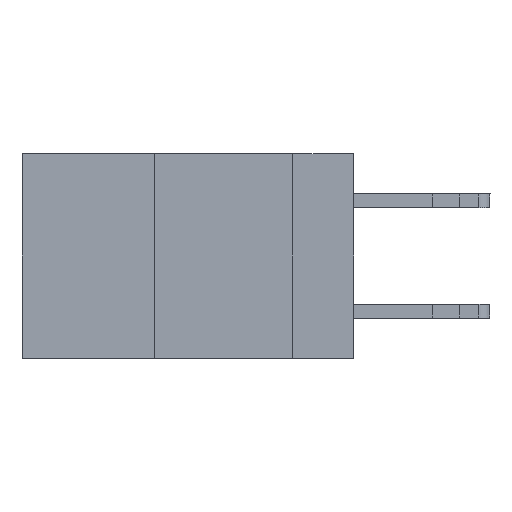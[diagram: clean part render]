
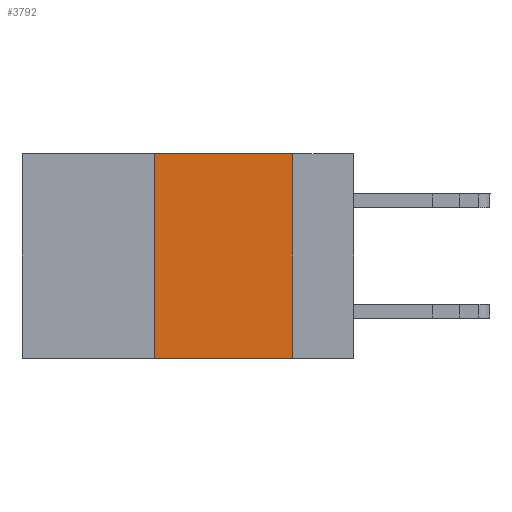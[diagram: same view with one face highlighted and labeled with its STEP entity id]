
A CAD part, left-side view. The second image highlights one B-rep face of the part: STEP entity #3792.
In plain terms, the highlighted planar face has unit normal (-1, 0, 0).
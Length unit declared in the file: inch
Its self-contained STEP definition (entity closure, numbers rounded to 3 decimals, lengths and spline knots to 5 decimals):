
#47 = ORIENTED_EDGE ( 'NONE', *, *, #14907, .T. ) ;
#554 = CARTESIAN_POINT ( 'NONE',  ( 0., 0.36, -0.37 ) ) ;
#1004 = CARTESIAN_POINT ( 'NONE',  ( 0., 0.6, -0.37 ) ) ;
#1065 = VECTOR ( 'NONE', #13622, 39.37008 ) ;
#1487 = DIRECTION ( 'NONE',  ( 0., -1., 0. ) ) ;
#2395 = CARTESIAN_POINT ( 'NONE',  ( 0., 0.6, 0. ) ) ;
#2685 = FACE_OUTER_BOUND ( 'NONE', #14182, .T. ) ;
#3030 = EDGE_CURVE ( 'NONE', #3723, #9920, #15404, .T. ) ;
#3723 = VERTEX_POINT ( 'NONE', #554 ) ;
#3792 = ADVANCED_FACE ( 'NONE', ( #2685 ), #3929, .F. ) ;
#3929 = PLANE ( 'NONE',  #10517 ) ;
#4660 = ORIENTED_EDGE ( 'NONE', *, *, #3030, .F. ) ;
#4810 = LINE ( 'NONE', #5394, #9489 ) ;
#5394 = CARTESIAN_POINT ( 'NONE',  ( 0., 0.11, 0. ) ) ;
#5586 = DIRECTION ( 'NONE',  ( 0., 0., -1. ) ) ;
#7175 = DIRECTION ( 'NONE',  ( 1., 0., 0. ) ) ;
#8979 = CARTESIAN_POINT ( 'NONE',  ( 0., 0.36, 0. ) ) ;
#9489 = VECTOR ( 'NONE', #19472, 39.37008 ) ;
#9553 = EDGE_CURVE ( 'NONE', #17729, #17404, #4810, .T. ) ;
#9920 = VERTEX_POINT ( 'NONE', #19717 ) ;
#10517 = AXIS2_PLACEMENT_3D ( 'NONE', #2395, #7175, #5586 ) ;
#11142 = VECTOR ( 'NONE', #15191, 39.37008 ) ;
#12611 = CARTESIAN_POINT ( 'NONE',  ( 0., 0.6, 0. ) ) ;
#13219 = EDGE_CURVE ( 'NONE', #9920, #17729, #15350, .T. ) ;
#13622 = DIRECTION ( 'NONE',  ( 0., -1., 0. ) ) ;
#14182 = EDGE_LOOP ( 'NONE', ( #15876, #19335, #4660, #47 ) ) ;
#14536 = CARTESIAN_POINT ( 'NONE',  ( 0., 0.11, 0. ) ) ;
#14902 = CARTESIAN_POINT ( 'NONE',  ( 0., 0.11, -0.37 ) ) ;
#14907 = EDGE_CURVE ( 'NONE', #3723, #17404, #18219, .T. ) ;
#15191 = DIRECTION ( 'NONE',  ( 0., 0., 1. ) ) ;
#15350 = LINE ( 'NONE', #12611, #19290 ) ;
#15404 = LINE ( 'NONE', #8979, #11142 ) ;
#15876 = ORIENTED_EDGE ( 'NONE', *, *, #9553, .F. ) ;
#17404 = VERTEX_POINT ( 'NONE', #14902 ) ;
#17729 = VERTEX_POINT ( 'NONE', #14536 ) ;
#18219 = LINE ( 'NONE', #1004, #1065 ) ;
#19290 = VECTOR ( 'NONE', #1487, 39.37008 ) ;
#19335 = ORIENTED_EDGE ( 'NONE', *, *, #13219, .F. ) ;
#19472 = DIRECTION ( 'NONE',  ( 0., 0., -1. ) ) ;
#19717 = CARTESIAN_POINT ( 'NONE',  ( 0., 0.36, 0. ) ) ;
